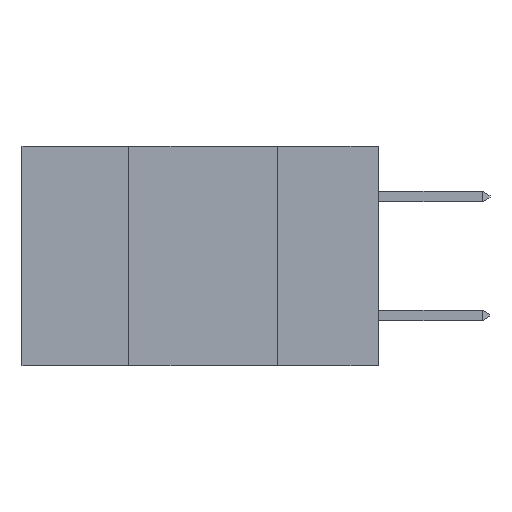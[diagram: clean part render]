
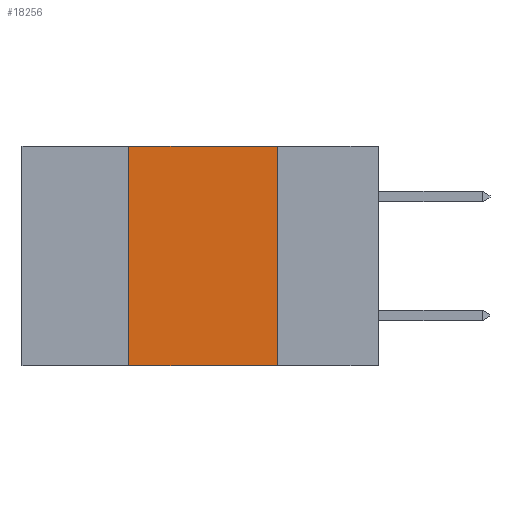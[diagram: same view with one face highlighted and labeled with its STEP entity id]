
A CAD part, left-side view. The second image highlights one B-rep face of the part: STEP entity #18256.
In plain terms, the highlighted planar face has unit normal (-1, 0, 0).
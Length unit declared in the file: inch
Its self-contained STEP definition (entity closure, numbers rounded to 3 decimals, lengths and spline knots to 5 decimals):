
#105 = VECTOR ( 'NONE', #9310, 39.37008 ) ;
#800 = CARTESIAN_POINT ( 'NONE',  ( 0., 0.17, -0.37 ) ) ;
#1462 = LINE ( 'NONE', #5685, #10548 ) ;
#2931 = VERTEX_POINT ( 'NONE', #14413 ) ;
#3157 = FACE_OUTER_BOUND ( 'NONE', #22537, .T. ) ;
#4471 = CARTESIAN_POINT ( 'NONE',  ( 0., 0.6, 0. ) ) ;
#4943 = LINE ( 'NONE', #16471, #105 ) ;
#5685 = CARTESIAN_POINT ( 'NONE',  ( 0., 0.42, 0. ) ) ;
#6259 = DIRECTION ( 'NONE',  ( 0., 0., -1. ) ) ;
#6870 = EDGE_CURVE ( 'NONE', #18774, #16334, #8916, .T. ) ;
#8916 = LINE ( 'NONE', #15814, #22504 ) ;
#9079 = AXIS2_PLACEMENT_3D ( 'NONE', #4471, #17046, #6259 ) ;
#9162 = LINE ( 'NONE', #15003, #18122 ) ;
#9310 = DIRECTION ( 'NONE',  ( 0., 0., -1. ) ) ;
#10548 = VECTOR ( 'NONE', #12942, 39.37008 ) ;
#11700 = ORIENTED_EDGE ( 'NONE', *, *, #16891, .F. ) ;
#11922 = VERTEX_POINT ( 'NONE', #21702 ) ;
#12856 = ORIENTED_EDGE ( 'NONE', *, *, #16803, .F. ) ;
#12942 = DIRECTION ( 'NONE',  ( 0., 0., 1. ) ) ;
#14343 = CARTESIAN_POINT ( 'NONE',  ( 0., 0.42, -0.37 ) ) ;
#14413 = CARTESIAN_POINT ( 'NONE',  ( 0., 0.17, 0. ) ) ;
#14772 = ORIENTED_EDGE ( 'NONE', *, *, #18855, .F. ) ;
#15003 = CARTESIAN_POINT ( 'NONE',  ( 0., 0.6, 0. ) ) ;
#15262 = PLANE ( 'NONE',  #9079 ) ;
#15814 = CARTESIAN_POINT ( 'NONE',  ( 0., 0.6, -0.37 ) ) ;
#16334 = VERTEX_POINT ( 'NONE', #800 ) ;
#16471 = CARTESIAN_POINT ( 'NONE',  ( 0., 0.17, 0. ) ) ;
#16758 = DIRECTION ( 'NONE',  ( 0., -1., 0. ) ) ;
#16803 = EDGE_CURVE ( 'NONE', #18774, #11922, #1462, .T. ) ;
#16808 = DIRECTION ( 'NONE',  ( 0., -1., 0. ) ) ;
#16891 = EDGE_CURVE ( 'NONE', #11922, #2931, #9162, .T. ) ;
#17046 = DIRECTION ( 'NONE',  ( 1., 0., 0. ) ) ;
#18122 = VECTOR ( 'NONE', #16808, 39.37008 ) ;
#18256 = ADVANCED_FACE ( 'NONE', ( #3157 ), #15262, .F. ) ;
#18774 = VERTEX_POINT ( 'NONE', #14343 ) ;
#18855 = EDGE_CURVE ( 'NONE', #2931, #16334, #4943, .T. ) ;
#20888 = ORIENTED_EDGE ( 'NONE', *, *, #6870, .T. ) ;
#21702 = CARTESIAN_POINT ( 'NONE',  ( 0., 0.42, 0. ) ) ;
#22504 = VECTOR ( 'NONE', #16758, 39.37008 ) ;
#22537 = EDGE_LOOP ( 'NONE', ( #14772, #11700, #12856, #20888 ) ) ;
